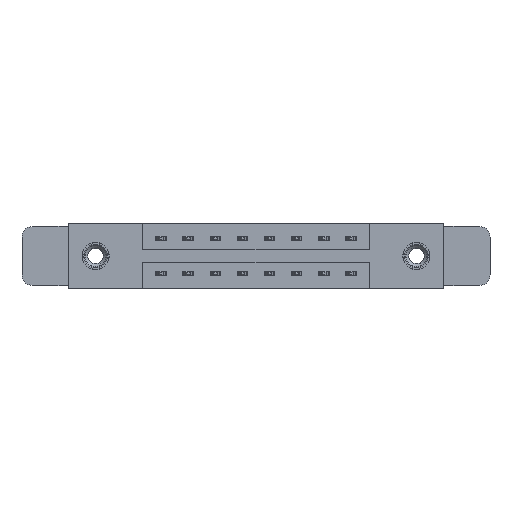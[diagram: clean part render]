
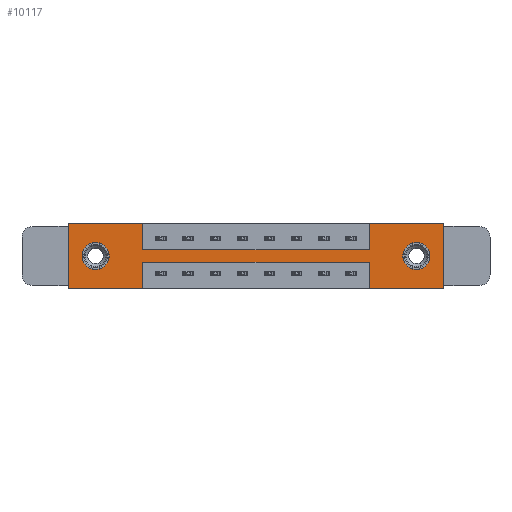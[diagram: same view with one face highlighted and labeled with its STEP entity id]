
A CAD part, front view. The second image highlights one B-rep face of the part: STEP entity #10117.
In plain terms, the highlighted planar face has unit normal (0, -1, 0).
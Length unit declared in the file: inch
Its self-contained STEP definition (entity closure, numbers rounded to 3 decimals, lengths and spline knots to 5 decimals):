
#80 = ORIENTED_EDGE ( 'NONE', *, *, #4926, .F. ) ;
#187 = VERTEX_POINT ( 'NONE', #12662 ) ;
#550 = VECTOR ( 'NONE', #789, 39.37008 ) ;
#652 = EDGE_CURVE ( 'NONE', #12006, #13090, #8104, .T. ) ;
#789 = DIRECTION ( 'NONE',  ( 1., 0., 0. ) ) ;
#889 = CARTESIAN_POINT ( 'NONE',  ( 1.999, 0., -0.107 ) ) ;
#974 = EDGE_LOOP ( 'NONE', ( #8917, #9023, #4299, #7334, #80, #7557, #3444, #1861, #5523, #3842, #5566, #11141 ) ) ;
#999 = EDGE_CURVE ( 'NONE', #4315, #5380, #1369, .T. ) ;
#1149 = DIRECTION ( 'NONE',  ( 0., 0., -1. ) ) ;
#1278 = LINE ( 'NONE', #11088, #8829 ) ;
#1369 = LINE ( 'NONE', #12981, #11459 ) ;
#1458 = CARTESIAN_POINT ( 'NONE',  ( 0., 0., -0.37 ) ) ;
#1571 = LINE ( 'NONE', #2107, #3972 ) ;
#1594 = PLANE ( 'NONE',  #9034 ) ;
#1642 = VERTEX_POINT ( 'NONE', #1740 ) ;
#1740 = CARTESIAN_POINT ( 'NONE',  ( 1.729, 0., -0.37 ) ) ;
#1861 = ORIENTED_EDGE ( 'NONE', *, *, #6177, .F. ) ;
#2107 = CARTESIAN_POINT ( 'NONE',  ( 2.154, 0., 0. ) ) ;
#2254 = EDGE_CURVE ( 'NONE', #1642, #10356, #6654, .T. ) ;
#2410 = LINE ( 'NONE', #12426, #10755 ) ;
#2546 = CARTESIAN_POINT ( 'NONE',  ( 1.729, 0., -0.22 ) ) ;
#2744 = CARTESIAN_POINT ( 'NONE',  ( 0., 0., 0. ) ) ;
#2821 = CIRCLE ( 'NONE', #3616, 0.078 ) ;
#3006 = LINE ( 'NONE', #8641, #6056 ) ;
#3116 = AXIS2_PLACEMENT_3D ( 'NONE', #13253, #4006, #11217 ) ;
#3359 = FACE_OUTER_BOUND ( 'NONE', #974, .T. ) ;
#3444 = ORIENTED_EDGE ( 'NONE', *, *, #8953, .F. ) ;
#3465 = CARTESIAN_POINT ( 'NONE',  ( 0.155, 0., -0.107 ) ) ;
#3616 = AXIS2_PLACEMENT_3D ( 'NONE', #10809, #11828, #12849 ) ;
#3620 = EDGE_CURVE ( 'NONE', #187, #1642, #4028, .T. ) ;
#3669 = DIRECTION ( 'NONE',  ( 0., 0., -1. ) ) ;
#3842 = ORIENTED_EDGE ( 'NONE', *, *, #6050, .F. ) ;
#3928 = VERTEX_POINT ( 'NONE', #9542 ) ;
#3957 = CARTESIAN_POINT ( 'NONE',  ( 1.999, 0., -0.185 ) ) ;
#3972 = VECTOR ( 'NONE', #1149, 39.37008 ) ;
#4006 = DIRECTION ( 'NONE',  ( 0., 1., 0. ) ) ;
#4009 = CARTESIAN_POINT ( 'NONE',  ( 0., 0., -0.37 ) ) ;
#4028 = LINE ( 'NONE', #4009, #10426 ) ;
#4052 = EDGE_CURVE ( 'NONE', #10356, #10722, #11035, .T. ) ;
#4283 = CIRCLE ( 'NONE', #7359, 0.078 ) ;
#4299 = ORIENTED_EDGE ( 'NONE', *, *, #2254, .F. ) ;
#4315 = VERTEX_POINT ( 'NONE', #9217 ) ;
#4557 = DIRECTION ( 'NONE',  ( 1., 0., 0. ) ) ;
#4650 = CARTESIAN_POINT ( 'NONE',  ( 1.729, 0., -0.37 ) ) ;
#4727 = VECTOR ( 'NONE', #4732, 39.37008 ) ;
#4732 = DIRECTION ( 'NONE',  ( 0., 0., 1. ) ) ;
#4926 = EDGE_CURVE ( 'NONE', #5380, #187, #1571, .T. ) ;
#5208 = CARTESIAN_POINT ( 'NONE',  ( 0.425, 0., -0.15 ) ) ;
#5380 = VERTEX_POINT ( 'NONE', #6111 ) ;
#5466 = CARTESIAN_POINT ( 'NONE',  ( 0., 0., 0. ) ) ;
#5523 = ORIENTED_EDGE ( 'NONE', *, *, #12041, .F. ) ;
#5566 = ORIENTED_EDGE ( 'NONE', *, *, #12607, .F. ) ;
#5679 = VERTEX_POINT ( 'NONE', #5713 ) ;
#5713 = CARTESIAN_POINT ( 'NONE',  ( 1.999, 0., -0.263 ) ) ;
#5781 = EDGE_CURVE ( 'NONE', #9635, #5679, #4283, .T. ) ;
#5798 = ORIENTED_EDGE ( 'NONE', *, *, #652, .T. ) ;
#5998 = EDGE_CURVE ( 'NONE', #5679, #9635, #2821, .T. ) ;
#6040 = LINE ( 'NONE', #2744, #550 ) ;
#6050 = EDGE_CURVE ( 'NONE', #8312, #3928, #6040, .T. ) ;
#6056 = VECTOR ( 'NONE', #9662, 39.37008 ) ;
#6111 = CARTESIAN_POINT ( 'NONE',  ( 2.154, 0., 0. ) ) ;
#6177 = EDGE_CURVE ( 'NONE', #10824, #12310, #6685, .T. ) ;
#6304 = DIRECTION ( 'NONE',  ( 0., 0., -1. ) ) ;
#6654 = LINE ( 'NONE', #4650, #4727 ) ;
#6685 = LINE ( 'NONE', #12913, #11465 ) ;
#6706 = CARTESIAN_POINT ( 'NONE',  ( 0.425, 0., -0.22 ) ) ;
#6738 = EDGE_LOOP ( 'NONE', ( #5798, #8237 ) ) ;
#6795 = DIRECTION ( 'NONE',  ( 1., 0., 0. ) ) ;
#7246 = DIRECTION ( 'NONE',  ( -1., 0., 0. ) ) ;
#7334 = ORIENTED_EDGE ( 'NONE', *, *, #3620, .F. ) ;
#7359 = AXIS2_PLACEMENT_3D ( 'NONE', #3957, #13073, #11116 ) ;
#7557 = ORIENTED_EDGE ( 'NONE', *, *, #999, .F. ) ;
#7682 = DIRECTION ( 'NONE',  ( 0., 1., 0. ) ) ;
#8039 = CARTESIAN_POINT ( 'NONE',  ( 1.729, 0., -0.15 ) ) ;
#8104 = CIRCLE ( 'NONE', #10051, 0.078 ) ;
#8237 = ORIENTED_EDGE ( 'NONE', *, *, #12375, .T. ) ;
#8312 = VERTEX_POINT ( 'NONE', #5466 ) ;
#8458 = CARTESIAN_POINT ( 'NONE',  ( 0.425, 0., -0.37 ) ) ;
#8641 = CARTESIAN_POINT ( 'NONE',  ( 0.425, 0., 0. ) ) ;
#8829 = VECTOR ( 'NONE', #9076, 39.37008 ) ;
#8917 = ORIENTED_EDGE ( 'NONE', *, *, #9010, .F. ) ;
#8953 = EDGE_CURVE ( 'NONE', #12310, #4315, #1278, .T. ) ;
#9010 = EDGE_CURVE ( 'NONE', #10722, #10109, #2410, .T. ) ;
#9023 = ORIENTED_EDGE ( 'NONE', *, *, #4052, .F. ) ;
#9034 = AXIS2_PLACEMENT_3D ( 'NONE', #1458, #9660, #3669 ) ;
#9076 = DIRECTION ( 'NONE',  ( 0., 0., 1. ) ) ;
#9217 = CARTESIAN_POINT ( 'NONE',  ( 1.729, 0., 0. ) ) ;
#9362 = CARTESIAN_POINT ( 'NONE',  ( 0.155, 0., -0.263 ) ) ;
#9542 = CARTESIAN_POINT ( 'NONE',  ( 0.425, 0., 0. ) ) ;
#9561 = LINE ( 'NONE', #10535, #12432 ) ;
#9597 = CARTESIAN_POINT ( 'NONE',  ( 0.155, 0., -0.185 ) ) ;
#9635 = VERTEX_POINT ( 'NONE', #889 ) ;
#9660 = DIRECTION ( 'NONE',  ( 0., -1., 0. ) ) ;
#9662 = DIRECTION ( 'NONE',  ( 0., 0., -1. ) ) ;
#9675 = CARTESIAN_POINT ( 'NONE',  ( 0., 0., -0.37 ) ) ;
#10038 = CIRCLE ( 'NONE', #3116, 0.078 ) ;
#10051 = AXIS2_PLACEMENT_3D ( 'NONE', #9597, #7682, #10719 ) ;
#10109 = VERTEX_POINT ( 'NONE', #8458 ) ;
#10117 = ADVANCED_FACE ( 'NONE', ( #11352, #11520, #3359 ), #1594, .T. ) ;
#10162 = DIRECTION ( 'NONE',  ( -1., 0., 0. ) ) ;
#10181 = LINE ( 'NONE', #11148, #12264 ) ;
#10356 = VERTEX_POINT ( 'NONE', #2546 ) ;
#10426 = VECTOR ( 'NONE', #7246, 39.37008 ) ;
#10524 = EDGE_LOOP ( 'NONE', ( #10750, #12608 ) ) ;
#10535 = CARTESIAN_POINT ( 'NONE',  ( 0., 0., 0. ) ) ;
#10577 = DIRECTION ( 'NONE',  ( 0., 0., 1. ) ) ;
#10666 = DIRECTION ( 'NONE',  ( -1., 0., 0. ) ) ;
#10719 = DIRECTION ( 'NONE',  ( 0., 0., 1. ) ) ;
#10722 = VERTEX_POINT ( 'NONE', #6706 ) ;
#10750 = ORIENTED_EDGE ( 'NONE', *, *, #5781, .T. ) ;
#10755 = VECTOR ( 'NONE', #6304, 39.37008 ) ;
#10809 = CARTESIAN_POINT ( 'NONE',  ( 1.999, 0., -0.185 ) ) ;
#10824 = VERTEX_POINT ( 'NONE', #5208 ) ;
#11035 = LINE ( 'NONE', #11815, #12798 ) ;
#11088 = CARTESIAN_POINT ( 'NONE',  ( 1.729, 0., 0. ) ) ;
#11116 = DIRECTION ( 'NONE',  ( 0., 0., -1. ) ) ;
#11141 = ORIENTED_EDGE ( 'NONE', *, *, #12997, .F. ) ;
#11148 = CARTESIAN_POINT ( 'NONE',  ( 0., 0., -0.37 ) ) ;
#11217 = DIRECTION ( 'NONE',  ( 0., 0., 1. ) ) ;
#11352 = FACE_BOUND ( 'NONE', #10524, .T. ) ;
#11459 = VECTOR ( 'NONE', #4557, 39.37008 ) ;
#11465 = VECTOR ( 'NONE', #6795, 39.37008 ) ;
#11520 = FACE_BOUND ( 'NONE', #6738, .T. ) ;
#11815 = CARTESIAN_POINT ( 'NONE',  ( 0.425, 0., -0.22 ) ) ;
#11828 = DIRECTION ( 'NONE',  ( 0., 1., 0. ) ) ;
#11952 = VERTEX_POINT ( 'NONE', #9675 ) ;
#12006 = VERTEX_POINT ( 'NONE', #3465 ) ;
#12041 = EDGE_CURVE ( 'NONE', #3928, #10824, #3006, .T. ) ;
#12264 = VECTOR ( 'NONE', #10162, 39.37008 ) ;
#12310 = VERTEX_POINT ( 'NONE', #8039 ) ;
#12375 = EDGE_CURVE ( 'NONE', #13090, #12006, #10038, .T. ) ;
#12426 = CARTESIAN_POINT ( 'NONE',  ( 0.425, 0., -0.37 ) ) ;
#12432 = VECTOR ( 'NONE', #10577, 39.37008 ) ;
#12607 = EDGE_CURVE ( 'NONE', #11952, #8312, #9561, .T. ) ;
#12608 = ORIENTED_EDGE ( 'NONE', *, *, #5998, .T. ) ;
#12662 = CARTESIAN_POINT ( 'NONE',  ( 2.154, 0., -0.37 ) ) ;
#12798 = VECTOR ( 'NONE', #10666, 39.37008 ) ;
#12849 = DIRECTION ( 'NONE',  ( 0., 0., -1. ) ) ;
#12913 = CARTESIAN_POINT ( 'NONE',  ( 0.425, 0., -0.15 ) ) ;
#12981 = CARTESIAN_POINT ( 'NONE',  ( 0., 0., 0. ) ) ;
#12997 = EDGE_CURVE ( 'NONE', #10109, #11952, #10181, .T. ) ;
#13073 = DIRECTION ( 'NONE',  ( 0., 1., 0. ) ) ;
#13090 = VERTEX_POINT ( 'NONE', #9362 ) ;
#13253 = CARTESIAN_POINT ( 'NONE',  ( 0.155, 0., -0.185 ) ) ;
